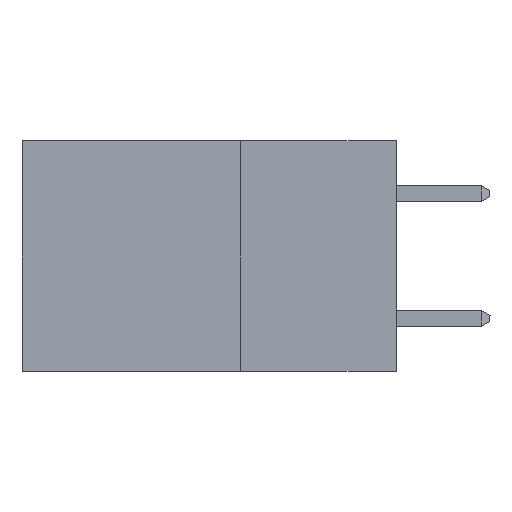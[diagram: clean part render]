
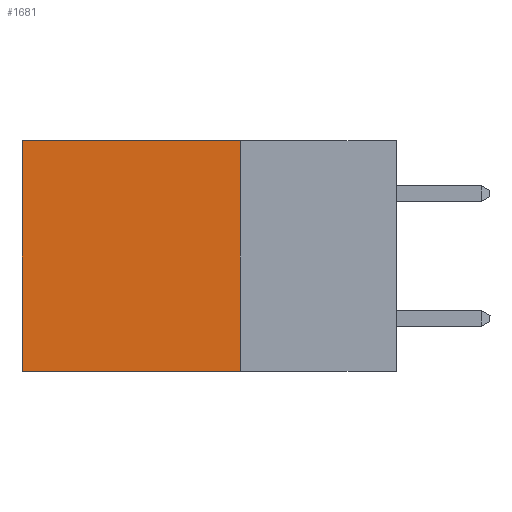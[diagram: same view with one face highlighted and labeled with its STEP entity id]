
A CAD part, left-side view. The second image highlights one B-rep face of the part: STEP entity #1681.
In plain terms, the highlighted planar face has unit normal (-1, 0, 0).
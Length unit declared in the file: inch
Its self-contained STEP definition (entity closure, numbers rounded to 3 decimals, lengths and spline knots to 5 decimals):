
#19 = CARTESIAN_POINT ( 'NONE',  ( 0.2615, 0.25, 0. ) ) ;
#61 = ORIENTED_EDGE ( 'NONE', *, *, #9382, .F. ) ;
#445 = VERTEX_POINT ( 'NONE', #6444 ) ;
#631 = VECTOR ( 'NONE', #5340, 39.37008 ) ;
#770 = ORIENTED_EDGE ( 'NONE', *, *, #1778, .T. ) ;
#1324 = DIRECTION ( 'NONE',  ( 1., 0., 0. ) ) ;
#1608 = DIRECTION ( 'NONE',  ( 0., 0., -1. ) ) ;
#1681 = ADVANCED_FACE ( 'NONE', ( #4363 ), #10652, .F. ) ;
#1778 = EDGE_CURVE ( 'NONE', #3636, #5205, #5630, .T. ) ;
#2476 = DIRECTION ( 'NONE',  ( 0., 0., -1. ) ) ;
#2536 = LINE ( 'NONE', #2940, #7092 ) ;
#2940 = CARTESIAN_POINT ( 'NONE',  ( 0.2615, 0.25, -0.37 ) ) ;
#3636 = VERTEX_POINT ( 'NONE', #19 ) ;
#4296 = CARTESIAN_POINT ( 'NONE',  ( 0.2615, 0.25, -0.37 ) ) ;
#4363 = FACE_OUTER_BOUND ( 'NONE', #7747, .T. ) ;
#5205 = VERTEX_POINT ( 'NONE', #6703 ) ;
#5340 = DIRECTION ( 'NONE',  ( 0., 0., -1. ) ) ;
#5593 = CARTESIAN_POINT ( 'NONE',  ( 0.2615, 0.6, -0.37 ) ) ;
#5630 = LINE ( 'NONE', #8984, #10146 ) ;
#6250 = ORIENTED_EDGE ( 'NONE', *, *, #9743, .F. ) ;
#6328 = EDGE_CURVE ( 'NONE', #5205, #445, #7757, .T. ) ;
#6444 = CARTESIAN_POINT ( 'NONE',  ( 0.2615, 0.6, -0.37 ) ) ;
#6616 = DIRECTION ( 'NONE',  ( 0., 1., 0. ) ) ;
#6703 = CARTESIAN_POINT ( 'NONE',  ( 0.2615, 0.6, 0. ) ) ;
#7092 = VECTOR ( 'NONE', #6616, 39.37008 ) ;
#7747 = EDGE_LOOP ( 'NONE', ( #9856, #6250, #61, #770 ) ) ;
#7757 = LINE ( 'NONE', #5593, #631 ) ;
#8510 = VERTEX_POINT ( 'NONE', #10247 ) ;
#8984 = CARTESIAN_POINT ( 'NONE',  ( 0.2615, 0.25, 0. ) ) ;
#9011 = DIRECTION ( 'NONE',  ( 0., 1., 0. ) ) ;
#9216 = LINE ( 'NONE', #4296, #11033 ) ;
#9382 = EDGE_CURVE ( 'NONE', #3636, #8510, #9216, .T. ) ;
#9504 = AXIS2_PLACEMENT_3D ( 'NONE', #10838, #1324, #2476 ) ;
#9743 = EDGE_CURVE ( 'NONE', #8510, #445, #2536, .T. ) ;
#9856 = ORIENTED_EDGE ( 'NONE', *, *, #6328, .T. ) ;
#10146 = VECTOR ( 'NONE', #9011, 39.37008 ) ;
#10247 = CARTESIAN_POINT ( 'NONE',  ( 0.2615, 0.25, -0.37 ) ) ;
#10652 = PLANE ( 'NONE',  #9504 ) ;
#10838 = CARTESIAN_POINT ( 'NONE',  ( 0.2615, 0.25, -0.37 ) ) ;
#11033 = VECTOR ( 'NONE', #1608, 39.37008 ) ;
